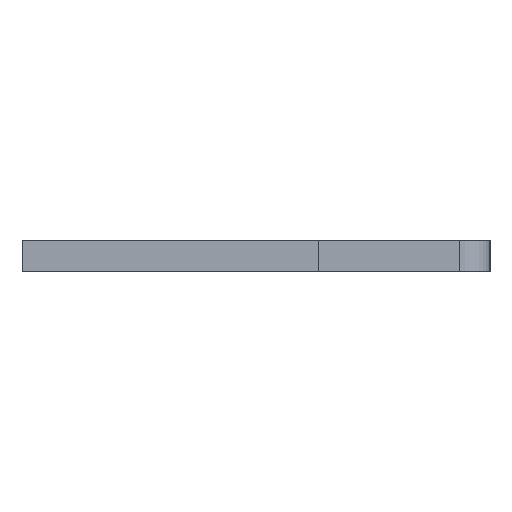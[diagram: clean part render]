
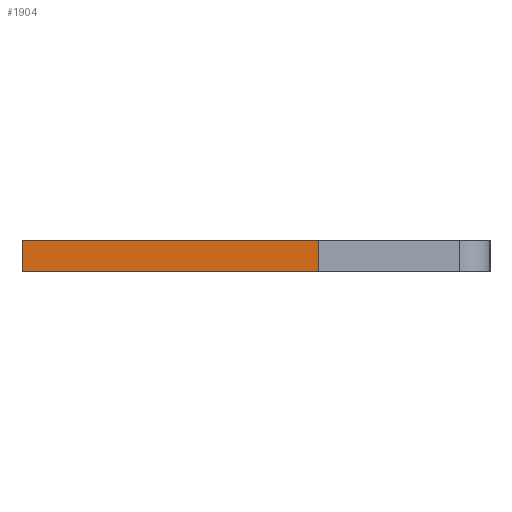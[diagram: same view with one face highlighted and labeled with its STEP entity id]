
A CAD part, left-side view. The second image highlights one B-rep face of the part: STEP entity #1904.
In plain terms, the highlighted face is planar.
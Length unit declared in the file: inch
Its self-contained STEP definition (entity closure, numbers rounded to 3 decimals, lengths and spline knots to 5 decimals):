
#365 = VERTEX_POINT ( 'NONE', #2214 ) ;
#481 = CARTESIAN_POINT ( 'NONE',  ( -0.01, 0.15, -0.04 ) ) ;
#713 = AXIS2_PLACEMENT_3D ( 'NONE', #1069, #2095, #2806 ) ;
#804 = VERTEX_POINT ( 'NONE', #1475 ) ;
#889 = LINE ( 'NONE', #2599, #1409 ) ;
#1059 = FACE_OUTER_BOUND ( 'NONE', #3077, .T. ) ;
#1069 = CARTESIAN_POINT ( 'NONE',  ( 0.01, 0.15, -0.04 ) ) ;
#1070 = ORIENTED_EDGE ( 'NONE', *, *, #1642, .T. ) ;
#1161 = ORIENTED_EDGE ( 'NONE', *, *, #2292, .F. ) ;
#1352 = VECTOR ( 'NONE', #2455, 39.37008 ) ;
#1396 = DIRECTION ( 'NONE',  ( 0., 1., 0. ) ) ;
#1409 = VECTOR ( 'NONE', #2407, 39.37008 ) ;
#1458 = CARTESIAN_POINT ( 'NONE',  ( 0.01, -0.04, -0.04 ) ) ;
#1475 = CARTESIAN_POINT ( 'NONE',  ( -0.01, -0.04, -0.04 ) ) ;
#1633 = CARTESIAN_POINT ( 'NONE',  ( -0.01, 0.15, -0.04 ) ) ;
#1642 = EDGE_CURVE ( 'NONE', #2981, #804, #3046, .T. ) ;
#1643 = VECTOR ( 'NONE', #2105, 39.37008 ) ;
#1850 = PLANE ( 'NONE',  #713 ) ;
#1887 = LINE ( 'NONE', #1633, #2892 ) ;
#1904 = ADVANCED_FACE ( 'NONE', ( #1059 ), #1850, .F. ) ;
#2095 = DIRECTION ( 'NONE',  ( 0., 0., 1. ) ) ;
#2105 = DIRECTION ( 'NONE',  ( -1., 0., 0. ) ) ;
#2198 = EDGE_CURVE ( 'NONE', #365, #2780, #2369, .T. ) ;
#2214 = CARTESIAN_POINT ( 'NONE',  ( 0.01, 0.15, -0.04 ) ) ;
#2292 = EDGE_CURVE ( 'NONE', #2981, #365, #889, .T. ) ;
#2369 = LINE ( 'NONE', #2857, #1643 ) ;
#2395 = EDGE_CURVE ( 'NONE', #804, #2780, #1887, .T. ) ;
#2407 = DIRECTION ( 'NONE',  ( 0., 1., 0. ) ) ;
#2455 = DIRECTION ( 'NONE',  ( -1., 0., 0. ) ) ;
#2599 = CARTESIAN_POINT ( 'NONE',  ( 0.01, 0.15, -0.04 ) ) ;
#2673 = CARTESIAN_POINT ( 'NONE',  ( 0.01, -0.04, -0.04 ) ) ;
#2780 = VERTEX_POINT ( 'NONE', #481 ) ;
#2788 = ORIENTED_EDGE ( 'NONE', *, *, #2198, .F. ) ;
#2806 = DIRECTION ( 'NONE',  ( 1., 0., 0. ) ) ;
#2855 = ORIENTED_EDGE ( 'NONE', *, *, #2395, .T. ) ;
#2857 = CARTESIAN_POINT ( 'NONE',  ( 0.01, 0.15, -0.04 ) ) ;
#2892 = VECTOR ( 'NONE', #1396, 39.37008 ) ;
#2981 = VERTEX_POINT ( 'NONE', #2673 ) ;
#3046 = LINE ( 'NONE', #1458, #1352 ) ;
#3077 = EDGE_LOOP ( 'NONE', ( #2855, #2788, #1161, #1070 ) ) ;
